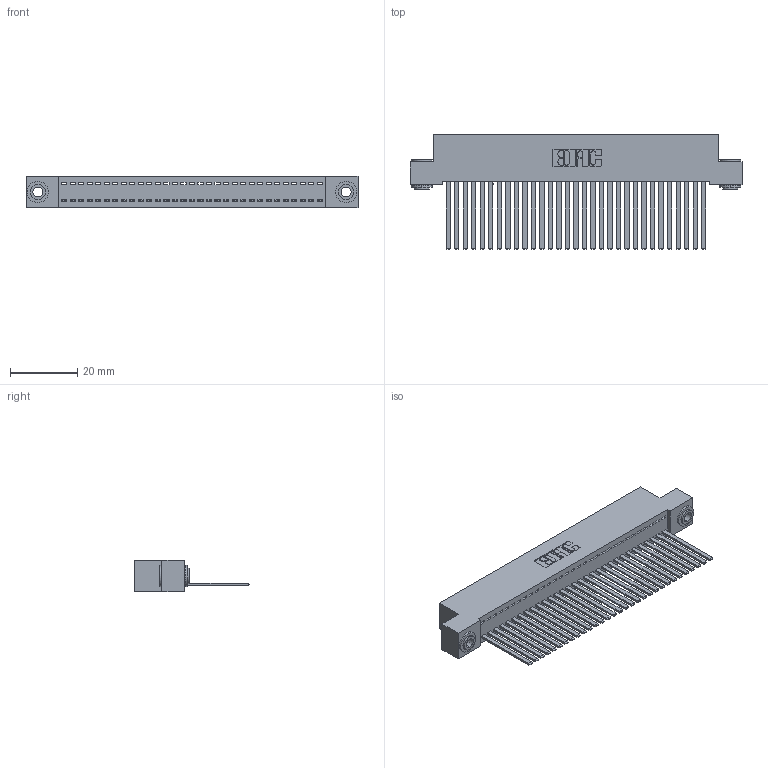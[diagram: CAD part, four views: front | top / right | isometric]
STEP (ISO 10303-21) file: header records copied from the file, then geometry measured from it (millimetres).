
FILE_DESCRIPTION (( 'STEP AP203' ), '1' );
FILE_NAME ('392-031-544-103.STEP', '2018-08-15T23:23:30', ( '' ), ( '' ), 'SwSTEP 2.0', 'SolidWorks 2016', '' );
FILE_SCHEMA (( 'CONFIG_CONTROL_DESIGN' ));
Length unit declared in the file: inch
Products named in the file (4): 342 Part_.156 TH; 345-292-001_345-293-144; 342-250-002_345-250-002-102; 392-031-544-103
Assembly tree (34 placements, depth 2):
  392-031-544-103
    342 Part_.156 TH
    345-292-001_345-293-144  x31
    342-250-002_345-250-002-102  x2
Bounding box: 99.06 x 34.3 x 9.4 mm (x, y, z)
Volume: 9026.9 mm3; surface area: 14298.2 mm2
Topology: 34 solids, 34 shells, 1760 faces, 5273 edges, 3470 vertices
Faces by surface type: plane 1254, cylinder 498, cone 8
Entity records: 20708 total; most frequent: CARTESIAN_POINT 3550, ORIENTED_EDGE 3510, DIRECTION 3047, EDGE_CURVE 1755, LINE 1607, VECTOR 1607, VERTEX_POINT 1166, AXIS2_PLACEMENT_3D 720
